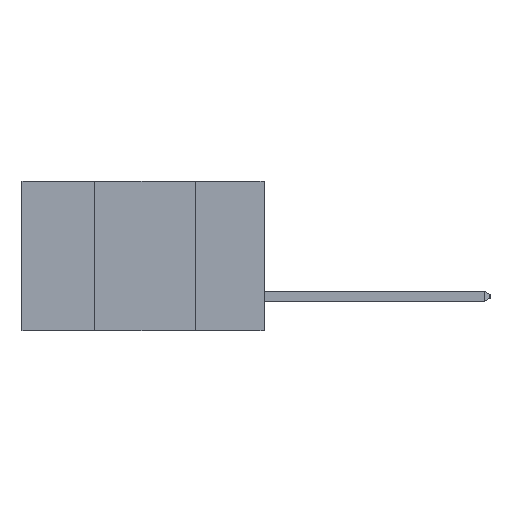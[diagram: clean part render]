
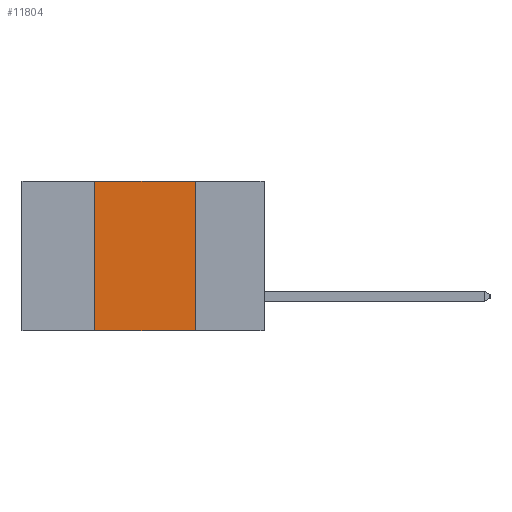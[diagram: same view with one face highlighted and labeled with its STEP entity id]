
A CAD part, left-side view. The second image highlights one B-rep face of the part: STEP entity #11804.
In plain terms, the highlighted planar face has unit normal (-1, 0, 0).
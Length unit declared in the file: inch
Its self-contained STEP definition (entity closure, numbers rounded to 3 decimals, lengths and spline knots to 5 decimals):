
#831 = LINE ( 'NONE', #10380, #11118 ) ;
#893 = VERTEX_POINT ( 'NONE', #5228 ) ;
#1084 = LINE ( 'NONE', #15894, #10978 ) ;
#1724 = DIRECTION ( 'NONE',  ( 0., 0., 1. ) ) ;
#2964 = EDGE_CURVE ( 'NONE', #893, #10629, #4572, .T. ) ;
#3560 = CARTESIAN_POINT ( 'NONE',  ( 0., 0.6, 0. ) ) ;
#3788 = VERTEX_POINT ( 'NONE', #10330 ) ;
#3815 = CARTESIAN_POINT ( 'NONE',  ( 0., 0.6, 0. ) ) ;
#4075 = CARTESIAN_POINT ( 'NONE',  ( 0., 0.17, -0.37 ) ) ;
#4153 = AXIS2_PLACEMENT_3D ( 'NONE', #3815, #5124, #14018 ) ;
#4572 = LINE ( 'NONE', #3560, #7607 ) ;
#4684 = EDGE_CURVE ( 'NONE', #10629, #6850, #1084, .T. ) ;
#5100 = CARTESIAN_POINT ( 'NONE',  ( 0., 0.17, 0. ) ) ;
#5124 = DIRECTION ( 'NONE',  ( 1., 0., 0. ) ) ;
#5228 = CARTESIAN_POINT ( 'NONE',  ( 0., 0.42, 0. ) ) ;
#6167 = ORIENTED_EDGE ( 'NONE', *, *, #2964, .F. ) ;
#6484 = DIRECTION ( 'NONE',  ( 0., -1., 0. ) ) ;
#6579 = ORIENTED_EDGE ( 'NONE', *, *, #14380, .F. ) ;
#6850 = VERTEX_POINT ( 'NONE', #4075 ) ;
#7252 = FACE_OUTER_BOUND ( 'NONE', #15875, .T. ) ;
#7384 = ORIENTED_EDGE ( 'NONE', *, *, #13562, .T. ) ;
#7607 = VECTOR ( 'NONE', #10005, 39.37008 ) ;
#7664 = LINE ( 'NONE', #9442, #11086 ) ;
#8382 = DIRECTION ( 'NONE',  ( 0., 0., -1. ) ) ;
#9442 = CARTESIAN_POINT ( 'NONE',  ( 0., 0.42, -0.37 ) ) ;
#10005 = DIRECTION ( 'NONE',  ( 0., -1., 0. ) ) ;
#10330 = CARTESIAN_POINT ( 'NONE',  ( 0., 0.42, -0.37 ) ) ;
#10380 = CARTESIAN_POINT ( 'NONE',  ( 0., 0.6, -0.37 ) ) ;
#10629 = VERTEX_POINT ( 'NONE', #5100 ) ;
#10978 = VECTOR ( 'NONE', #8382, 39.37008 ) ;
#11086 = VECTOR ( 'NONE', #1724, 39.37008 ) ;
#11118 = VECTOR ( 'NONE', #6484, 39.37008 ) ;
#11804 = ADVANCED_FACE ( 'NONE', ( #7252 ), #12797, .F. ) ;
#12797 = PLANE ( 'NONE',  #4153 ) ;
#13562 = EDGE_CURVE ( 'NONE', #3788, #6850, #831, .T. ) ;
#14018 = DIRECTION ( 'NONE',  ( 0., 0., -1. ) ) ;
#14380 = EDGE_CURVE ( 'NONE', #3788, #893, #7664, .T. ) ;
#15795 = ORIENTED_EDGE ( 'NONE', *, *, #4684, .F. ) ;
#15875 = EDGE_LOOP ( 'NONE', ( #15795, #6167, #6579, #7384 ) ) ;
#15894 = CARTESIAN_POINT ( 'NONE',  ( 0., 0.17, -0.37 ) ) ;
